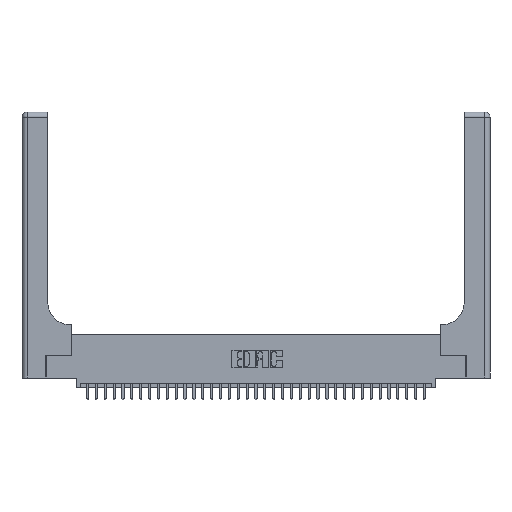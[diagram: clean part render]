
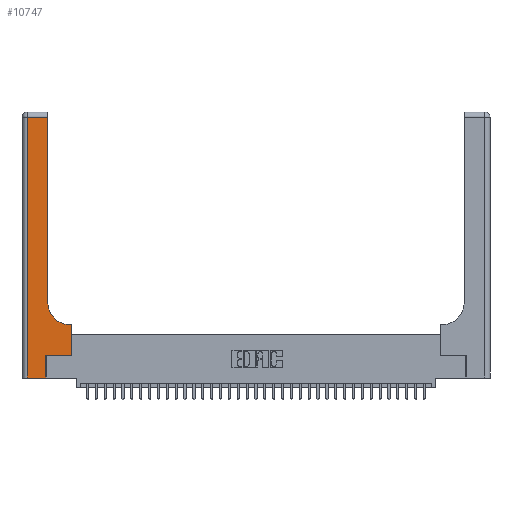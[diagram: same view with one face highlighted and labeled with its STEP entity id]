
A CAD part, top view. The second image highlights one B-rep face of the part: STEP entity #10747.
In plain terms, the highlighted planar face has unit normal (0, 0, 1).
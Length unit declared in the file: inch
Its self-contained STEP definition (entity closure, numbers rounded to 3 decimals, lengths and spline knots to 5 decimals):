
#212 = LINE ( 'NONE', #20216, #14460 ) ;
#718 = AXIS2_PLACEMENT_3D ( 'NONE', #5630, #25284, #8472 ) ;
#944 = DIRECTION ( 'NONE',  ( 1., 0., 0. ) ) ;
#1005 = EDGE_CURVE ( 'NONE', #5722, #23922, #212, .T. ) ;
#1030 = CARTESIAN_POINT ( 'NONE',  ( 0.269, 0., 0.37 ) ) ;
#1253 = CARTESIAN_POINT ( 'NONE',  ( 0.2915, 0.85, 0.37 ) ) ;
#1590 = VECTOR ( 'NONE', #11703, 39.37008 ) ;
#1775 = ORIENTED_EDGE ( 'NONE', *, *, #1005, .T. ) ;
#1934 = CARTESIAN_POINT ( 'NONE',  ( 0.06, 2.94, 0.37 ) ) ;
#2592 = CARTESIAN_POINT ( 'NONE',  ( 0.5415, 0.6, 0.37 ) ) ;
#3502 = DIRECTION ( 'NONE',  ( -1., 0., 0. ) ) ;
#3712 = CARTESIAN_POINT ( 'NONE',  ( 0.5585, 0.6, 0.37 ) ) ;
#4622 = CARTESIAN_POINT ( 'NONE',  ( 0.2915, 2.94, 0.37 ) ) ;
#5285 = CARTESIAN_POINT ( 'NONE',  ( 0.2915, 3., 0.37 ) ) ;
#5630 = CARTESIAN_POINT ( 'NONE',  ( 0.5415, 0.85, 0.37 ) ) ;
#5722 = VERTEX_POINT ( 'NONE', #35132 ) ;
#5891 = DIRECTION ( 'NONE',  ( -1., 0., 0. ) ) ;
#6336 = LINE ( 'NONE', #5285, #12958 ) ;
#6521 = LINE ( 'NONE', #11575, #19754 ) ;
#7083 = EDGE_CURVE ( 'NONE', #27320, #21124, #25437, .T. ) ;
#8069 = PLANE ( 'NONE',  #35350 ) ;
#8107 = DIRECTION ( 'NONE',  ( 0., 1., 0. ) ) ;
#8472 = DIRECTION ( 'NONE',  ( 1., 0., 0. ) ) ;
#8748 = CARTESIAN_POINT ( 'NONE',  ( 0.06, 3., 0.37 ) ) ;
#8896 = CIRCLE ( 'NONE', #718, 0.25 ) ;
#9167 = LINE ( 'NONE', #8748, #1590 ) ;
#9636 = CARTESIAN_POINT ( 'NONE',  ( 0.269, 0.25, 0.37 ) ) ;
#9698 = VECTOR ( 'NONE', #944, 39.37008 ) ;
#10747 = ADVANCED_FACE ( 'NONE', ( #33537 ), #8069, .F. ) ;
#10924 = DIRECTION ( 'NONE',  ( 0., 0., -1. ) ) ;
#11279 = VERTEX_POINT ( 'NONE', #1934 ) ;
#11575 = CARTESIAN_POINT ( 'NONE',  ( 0., 2.94, 0.37 ) ) ;
#11703 = DIRECTION ( 'NONE',  ( 0., -1., 0. ) ) ;
#12512 = LINE ( 'NONE', #14822, #33892 ) ;
#12787 = ORIENTED_EDGE ( 'NONE', *, *, #32128, .T. ) ;
#12935 = EDGE_CURVE ( 'NONE', #21124, #5722, #16021, .T. ) ;
#12958 = VECTOR ( 'NONE', #8107, 39.37008 ) ;
#13950 = ORIENTED_EDGE ( 'NONE', *, *, #32401, .T. ) ;
#14460 = VECTOR ( 'NONE', #31379, 39.37008 ) ;
#14822 = CARTESIAN_POINT ( 'NONE',  ( 0.2915, 0.6, 0.37 ) ) ;
#15746 = VERTEX_POINT ( 'NONE', #2592 ) ;
#16021 = LINE ( 'NONE', #20381, #29973 ) ;
#16085 = ORIENTED_EDGE ( 'NONE', *, *, #21572, .T. ) ;
#17207 = EDGE_CURVE ( 'NONE', #11279, #36315, #9167, .T. ) ;
#17415 = VERTEX_POINT ( 'NONE', #1253 ) ;
#17484 = ORIENTED_EDGE ( 'NONE', *, *, #28652, .T. ) ;
#17552 = DIRECTION ( 'NONE',  ( 1., 0., 0. ) ) ;
#19754 = VECTOR ( 'NONE', #5891, 39.37008 ) ;
#20216 = CARTESIAN_POINT ( 'NONE',  ( 0.5585, 0.25, 0.37 ) ) ;
#20381 = CARTESIAN_POINT ( 'NONE',  ( 0.269, 0.25, 0.37 ) ) ;
#21124 = VERTEX_POINT ( 'NONE', #9636 ) ;
#21572 = EDGE_CURVE ( 'NONE', #36359, #11279, #6521, .T. ) ;
#21752 = DIRECTION ( 'NONE',  ( 0., 1., 0. ) ) ;
#23922 = VERTEX_POINT ( 'NONE', #3712 ) ;
#24168 = CARTESIAN_POINT ( 'NONE',  ( 0.06, 0., 0.37 ) ) ;
#24615 = LINE ( 'NONE', #31781, #9698 ) ;
#24631 = ORIENTED_EDGE ( 'NONE', *, *, #17207, .T. ) ;
#25284 = DIRECTION ( 'NONE',  ( 0., 0., -1. ) ) ;
#25437 = LINE ( 'NONE', #35603, #31943 ) ;
#25864 = ORIENTED_EDGE ( 'NONE', *, *, #7083, .T. ) ;
#26626 = EDGE_LOOP ( 'NONE', ( #12787, #16085, #24631, #17484, #25864, #32625, #1775, #13950, #29799 ) ) ;
#27320 = VERTEX_POINT ( 'NONE', #1030 ) ;
#27688 = CARTESIAN_POINT ( 'NONE',  ( 0., 3., 0.37 ) ) ;
#28652 = EDGE_CURVE ( 'NONE', #36315, #27320, #24615, .T. ) ;
#29799 = ORIENTED_EDGE ( 'NONE', *, *, #35873, .T. ) ;
#29973 = VECTOR ( 'NONE', #17552, 39.37008 ) ;
#30494 = DIRECTION ( 'NONE',  ( -1., 0., 0. ) ) ;
#31379 = DIRECTION ( 'NONE',  ( 0., 1., 0. ) ) ;
#31781 = CARTESIAN_POINT ( 'NONE',  ( 0., 0., 0.37 ) ) ;
#31943 = VECTOR ( 'NONE', #21752, 39.37008 ) ;
#32128 = EDGE_CURVE ( 'NONE', #17415, #36359, #6336, .T. ) ;
#32401 = EDGE_CURVE ( 'NONE', #23922, #15746, #12512, .T. ) ;
#32625 = ORIENTED_EDGE ( 'NONE', *, *, #12935, .T. ) ;
#33537 = FACE_OUTER_BOUND ( 'NONE', #26626, .T. ) ;
#33892 = VECTOR ( 'NONE', #3502, 39.37008 ) ;
#35132 = CARTESIAN_POINT ( 'NONE',  ( 0.5585, 0.25, 0.37 ) ) ;
#35350 = AXIS2_PLACEMENT_3D ( 'NONE', #27688, #10924, #30494 ) ;
#35603 = CARTESIAN_POINT ( 'NONE',  ( 0.269, 0., 0.37 ) ) ;
#35873 = EDGE_CURVE ( 'NONE', #15746, #17415, #8896, .T. ) ;
#36315 = VERTEX_POINT ( 'NONE', #24168 ) ;
#36359 = VERTEX_POINT ( 'NONE', #4622 ) ;
